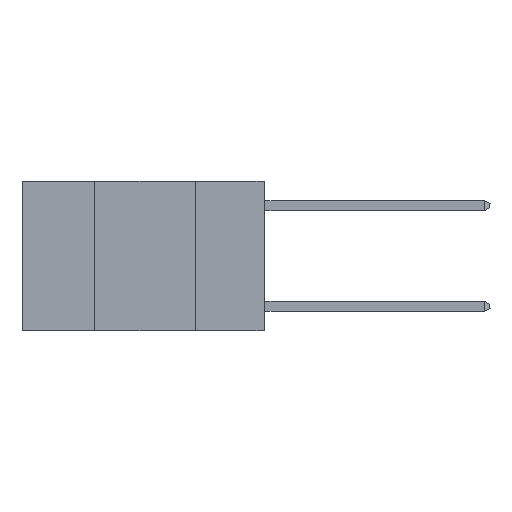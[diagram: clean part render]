
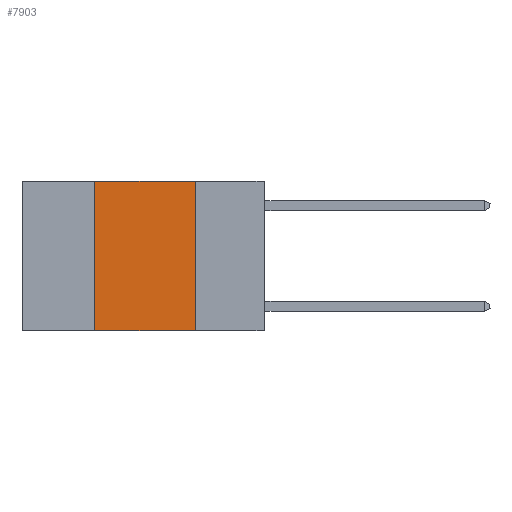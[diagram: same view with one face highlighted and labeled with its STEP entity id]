
A CAD part, left-side view. The second image highlights one B-rep face of the part: STEP entity #7903.
In plain terms, the highlighted planar face has unit normal (-1, 0, 0).
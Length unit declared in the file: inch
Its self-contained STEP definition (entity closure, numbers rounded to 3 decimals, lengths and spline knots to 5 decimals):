
#746 = VECTOR ( 'NONE', #1164, 39.37008 ) ;
#1164 = DIRECTION ( 'NONE',  ( 0., 0., 1. ) ) ;
#1507 = DIRECTION ( 'NONE',  ( 0., 0., -1. ) ) ;
#2241 = VERTEX_POINT ( 'NONE', #5560 ) ;
#3083 = EDGE_CURVE ( 'NONE', #2241, #11132, #17457, .T. ) ;
#3977 = LINE ( 'NONE', #17000, #8588 ) ;
#5183 = EDGE_LOOP ( 'NONE', ( #7746, #6487, #5544, #14097 ) ) ;
#5334 = CARTESIAN_POINT ( 'NONE',  ( 0., 0.17, 0. ) ) ;
#5544 = ORIENTED_EDGE ( 'NONE', *, *, #3083, .F. ) ;
#5560 = CARTESIAN_POINT ( 'NONE',  ( 0., 0.42, -0.37 ) ) ;
#5561 = AXIS2_PLACEMENT_3D ( 'NONE', #12213, #15487, #6578 ) ;
#6487 = ORIENTED_EDGE ( 'NONE', *, *, #16865, .F. ) ;
#6578 = DIRECTION ( 'NONE',  ( 0., 0., -1. ) ) ;
#7619 = VECTOR ( 'NONE', #1507, 39.37008 ) ;
#7746 = ORIENTED_EDGE ( 'NONE', *, *, #12156, .F. ) ;
#7894 = FACE_OUTER_BOUND ( 'NONE', #5183, .T. ) ;
#7903 = ADVANCED_FACE ( 'NONE', ( #7894 ), #16948, .F. ) ;
#8306 = DIRECTION ( 'NONE',  ( 0., -1., 0. ) ) ;
#8588 = VECTOR ( 'NONE', #8306, 39.37008 ) ;
#8622 = LINE ( 'NONE', #11143, #13492 ) ;
#8705 = CARTESIAN_POINT ( 'NONE',  ( 0., 0.17, -0.37 ) ) ;
#8711 = VERTEX_POINT ( 'NONE', #5334 ) ;
#11132 = VERTEX_POINT ( 'NONE', #15365 ) ;
#11143 = CARTESIAN_POINT ( 'NONE',  ( 0., 0.6, -0.37 ) ) ;
#11960 = CARTESIAN_POINT ( 'NONE',  ( 0., 0.42, 0. ) ) ;
#12156 = EDGE_CURVE ( 'NONE', #8711, #12171, #16127, .T. ) ;
#12171 = VERTEX_POINT ( 'NONE', #8705 ) ;
#12213 = CARTESIAN_POINT ( 'NONE',  ( 0., 0.6, 0. ) ) ;
#12941 = CARTESIAN_POINT ( 'NONE',  ( 0., 0.17, 0. ) ) ;
#13492 = VECTOR ( 'NONE', #17408, 39.37008 ) ;
#14097 = ORIENTED_EDGE ( 'NONE', *, *, #16060, .T. ) ;
#15365 = CARTESIAN_POINT ( 'NONE',  ( 0., 0.42, 0. ) ) ;
#15487 = DIRECTION ( 'NONE',  ( 1., 0., 0. ) ) ;
#16060 = EDGE_CURVE ( 'NONE', #2241, #12171, #8622, .T. ) ;
#16127 = LINE ( 'NONE', #12941, #7619 ) ;
#16865 = EDGE_CURVE ( 'NONE', #11132, #8711, #3977, .T. ) ;
#16948 = PLANE ( 'NONE',  #5561 ) ;
#17000 = CARTESIAN_POINT ( 'NONE',  ( 0., 0.6, 0. ) ) ;
#17408 = DIRECTION ( 'NONE',  ( 0., -1., 0. ) ) ;
#17457 = LINE ( 'NONE', #11960, #746 ) ;
